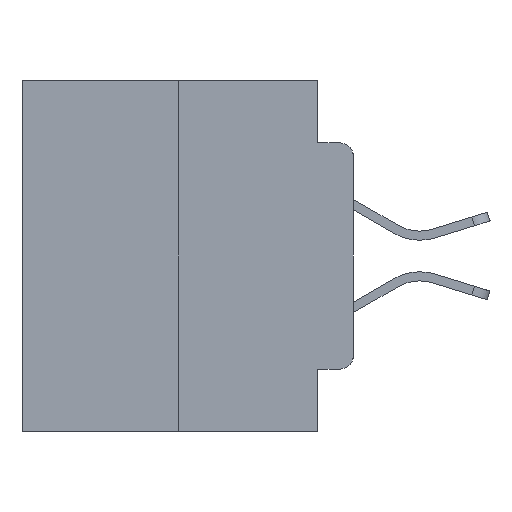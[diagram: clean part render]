
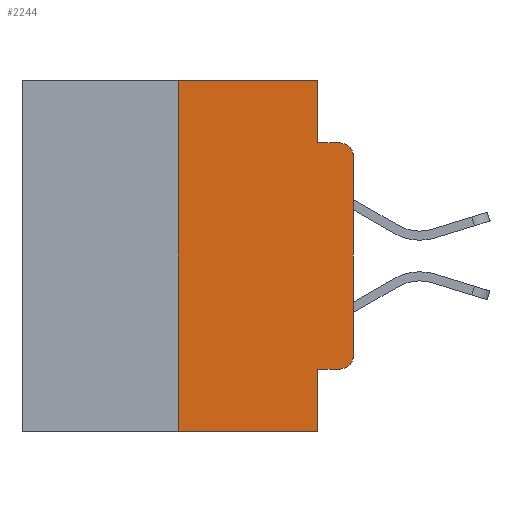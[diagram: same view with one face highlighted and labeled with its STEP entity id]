
A CAD part, left-side view. The second image highlights one B-rep face of the part: STEP entity #2244.
In plain terms, the highlighted planar face has unit normal (-1, 0, 0).
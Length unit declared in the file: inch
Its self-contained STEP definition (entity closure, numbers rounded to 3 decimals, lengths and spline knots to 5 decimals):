
#720 = LINE ( 'NONE', #8837, #13941 ) ;
#815 = EDGE_CURVE ( 'NONE', #5338, #13332, #1651, .T. ) ;
#907 = VECTOR ( 'NONE', #22806, 39.37008 ) ;
#965 = CIRCLE ( 'NONE', #10449, 0.02 ) ;
#1482 = VERTEX_POINT ( 'NONE', #17435 ) ;
#1584 = VERTEX_POINT ( 'NONE', #17040 ) ;
#1651 = LINE ( 'NONE', #22085, #11241 ) ;
#1695 = PLANE ( 'NONE',  #18097 ) ;
#1755 = EDGE_CURVE ( 'NONE', #5338, #1482, #24067, .T. ) ;
#1979 = CARTESIAN_POINT ( 'NONE',  ( 0., 0.051, -0.0885 ) ) ;
#2244 = ADVANCED_FACE ( 'NONE', ( #10457 ), #1695, .F. ) ;
#3383 = CARTESIAN_POINT ( 'NONE',  ( 0., 0.25, 0. ) ) ;
#3512 = EDGE_CURVE ( 'NONE', #26582, #1584, #16717, .T. ) ;
#3698 = EDGE_CURVE ( 'NONE', #1482, #5947, #720, .T. ) ;
#3717 = ORIENTED_EDGE ( 'NONE', *, *, #12351, .T. ) ;
#4027 = VECTOR ( 'NONE', #13758, 39.37008 ) ;
#4469 = ORIENTED_EDGE ( 'NONE', *, *, #1755, .F. ) ;
#4605 = VECTOR ( 'NONE', #25699, 39.37008 ) ;
#5151 = DIRECTION ( 'NONE',  ( -1., 0., 0. ) ) ;
#5338 = VERTEX_POINT ( 'NONE', #15510 ) ;
#5561 = CARTESIAN_POINT ( 'NONE',  ( 0., 0.051, -0.4115 ) ) ;
#5599 = LINE ( 'NONE', #26174, #11468 ) ;
#5705 = CARTESIAN_POINT ( 'NONE',  ( 0., 0.051, -0.4115 ) ) ;
#5947 = VERTEX_POINT ( 'NONE', #13710 ) ;
#5960 = EDGE_CURVE ( 'NONE', #10526, #21868, #23859, .T. ) ;
#6393 = DIRECTION ( 'NONE',  ( -1., 0., 0. ) ) ;
#7053 = EDGE_CURVE ( 'NONE', #5947, #26582, #8980, .T. ) ;
#7458 = DIRECTION ( 'NONE',  ( 0., -1., 0. ) ) ;
#8654 = ORIENTED_EDGE ( 'NONE', *, *, #3698, .F. ) ;
#8660 = CARTESIAN_POINT ( 'NONE',  ( 0., 0., 0. ) ) ;
#8837 = CARTESIAN_POINT ( 'NONE',  ( 0., 0.473, 0. ) ) ;
#8980 = LINE ( 'NONE', #17259, #20005 ) ;
#9181 = DIRECTION ( 'NONE',  ( 0., 0., -1. ) ) ;
#10379 = EDGE_CURVE ( 'NONE', #10782, #13332, #5599, .T. ) ;
#10449 = AXIS2_PLACEMENT_3D ( 'NONE', #12984, #5151, #9181 ) ;
#10457 = FACE_OUTER_BOUND ( 'NONE', #23849, .T. ) ;
#10526 = VERTEX_POINT ( 'NONE', #18590 ) ;
#10715 = ORIENTED_EDGE ( 'NONE', *, *, #3512, .F. ) ;
#10782 = VERTEX_POINT ( 'NONE', #5561 ) ;
#11241 = VECTOR ( 'NONE', #7458, 39.37008 ) ;
#11468 = VECTOR ( 'NONE', #26446, 39.37008 ) ;
#11690 = ORIENTED_EDGE ( 'NONE', *, *, #24127, .T. ) ;
#12104 = DIRECTION ( 'NONE',  ( 1., 0., 0. ) ) ;
#12127 = EDGE_CURVE ( 'NONE', #10782, #10526, #23850, .T. ) ;
#12351 = EDGE_CURVE ( 'NONE', #21868, #26644, #23673, .T. ) ;
#12984 = CARTESIAN_POINT ( 'NONE',  ( 0., 0.02, -0.1085 ) ) ;
#13162 = DIRECTION ( 'NONE',  ( 0., -1., 0. ) ) ;
#13332 = VERTEX_POINT ( 'NONE', #16312 ) ;
#13710 = CARTESIAN_POINT ( 'NONE',  ( 0., 0.051, 0. ) ) ;
#13758 = DIRECTION ( 'NONE',  ( 0., 0., 1. ) ) ;
#13941 = VECTOR ( 'NONE', #13162, 39.37008 ) ;
#14217 = CARTESIAN_POINT ( 'NONE',  ( 0., 0., -0.1085 ) ) ;
#15510 = CARTESIAN_POINT ( 'NONE',  ( 0., 0.25, -0.5 ) ) ;
#15562 = ORIENTED_EDGE ( 'NONE', *, *, #815, .T. ) ;
#16065 = AXIS2_PLACEMENT_3D ( 'NONE', #16694, #6393, #16419 ) ;
#16312 = CARTESIAN_POINT ( 'NONE',  ( 0., 0.051, -0.5 ) ) ;
#16419 = DIRECTION ( 'NONE',  ( 0., 0., -1. ) ) ;
#16694 = CARTESIAN_POINT ( 'NONE',  ( 0., 0.02, -0.3915 ) ) ;
#16717 = LINE ( 'NONE', #1979, #907 ) ;
#16731 = CARTESIAN_POINT ( 'NONE',  ( 0., 0., -0.3915 ) ) ;
#17040 = CARTESIAN_POINT ( 'NONE',  ( 0., 0.02, -0.0885 ) ) ;
#17259 = CARTESIAN_POINT ( 'NONE',  ( 0., 0.051, 0. ) ) ;
#17435 = CARTESIAN_POINT ( 'NONE',  ( 0., 0.25, 0. ) ) ;
#17891 = CARTESIAN_POINT ( 'NONE',  ( 0., 0.051, -0.0885 ) ) ;
#18097 = AXIS2_PLACEMENT_3D ( 'NONE', #26469, #12104, #18745 ) ;
#18590 = CARTESIAN_POINT ( 'NONE',  ( 0., 0.02, -0.4115 ) ) ;
#18745 = DIRECTION ( 'NONE',  ( 0., 0., -1. ) ) ;
#19690 = VECTOR ( 'NONE', #26013, 39.37008 ) ;
#20005 = VECTOR ( 'NONE', #25507, 39.37008 ) ;
#20151 = ORIENTED_EDGE ( 'NONE', *, *, #7053, .F. ) ;
#20704 = ORIENTED_EDGE ( 'NONE', *, *, #10379, .F. ) ;
#21653 = ORIENTED_EDGE ( 'NONE', *, *, #12127, .T. ) ;
#21868 = VERTEX_POINT ( 'NONE', #16731 ) ;
#22085 = CARTESIAN_POINT ( 'NONE',  ( 0., 0.473, -0.5 ) ) ;
#22685 = ORIENTED_EDGE ( 'NONE', *, *, #5960, .T. ) ;
#22806 = DIRECTION ( 'NONE',  ( 0., -1., 0. ) ) ;
#23673 = LINE ( 'NONE', #8660, #4605 ) ;
#23849 = EDGE_LOOP ( 'NONE', ( #3717, #11690, #10715, #20151, #8654, #4469, #15562, #20704, #21653, #22685 ) ) ;
#23850 = LINE ( 'NONE', #5705, #19690 ) ;
#23859 = CIRCLE ( 'NONE', #16065, 0.02 ) ;
#24067 = LINE ( 'NONE', #3383, #4027 ) ;
#24127 = EDGE_CURVE ( 'NONE', #26644, #1584, #965, .T. ) ;
#25507 = DIRECTION ( 'NONE',  ( 0., 0., -1. ) ) ;
#25699 = DIRECTION ( 'NONE',  ( 0., 0., 1. ) ) ;
#26013 = DIRECTION ( 'NONE',  ( 0., -1., 0. ) ) ;
#26174 = CARTESIAN_POINT ( 'NONE',  ( 0., 0.051, 0. ) ) ;
#26446 = DIRECTION ( 'NONE',  ( 0., 0., -1. ) ) ;
#26469 = CARTESIAN_POINT ( 'NONE',  ( 0., 0.473, 0. ) ) ;
#26582 = VERTEX_POINT ( 'NONE', #17891 ) ;
#26644 = VERTEX_POINT ( 'NONE', #14217 ) ;
